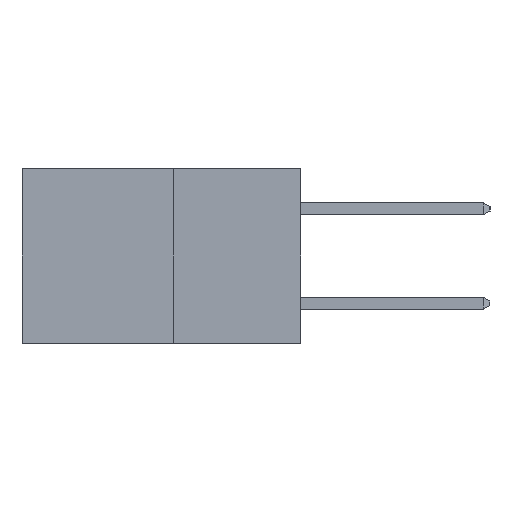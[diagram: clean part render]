
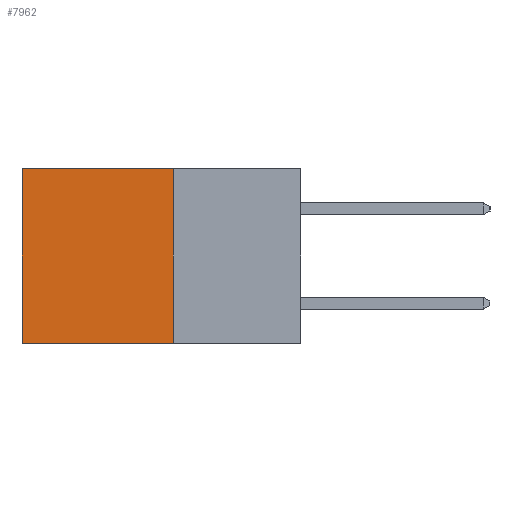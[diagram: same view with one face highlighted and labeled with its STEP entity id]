
A CAD part, left-side view. The second image highlights one B-rep face of the part: STEP entity #7962.
In plain terms, the highlighted planar face has unit normal (-1, 0, 0).
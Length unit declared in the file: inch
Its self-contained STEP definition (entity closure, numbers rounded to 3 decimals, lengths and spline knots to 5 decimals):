
#38 = VERTEX_POINT ( 'NONE', #3453 ) ;
#79 = DIRECTION ( 'NONE',  ( 0., 0., -1. ) ) ;
#374 = FACE_OUTER_BOUND ( 'NONE', #5023, .T. ) ;
#491 = VERTEX_POINT ( 'NONE', #4147 ) ;
#562 = DIRECTION ( 'NONE',  ( 1., 0., 0. ) ) ;
#1275 = VERTEX_POINT ( 'NONE', #5590 ) ;
#1349 = VECTOR ( 'NONE', #2227, 39.37008 ) ;
#1377 = DIRECTION ( 'NONE',  ( 0., 1., 0. ) ) ;
#1500 = CARTESIAN_POINT ( 'NONE',  ( 0.277, 0.27, -0.37 ) ) ;
#1899 = LINE ( 'NONE', #4761, #6907 ) ;
#2227 = DIRECTION ( 'NONE',  ( 0., 0., -1. ) ) ;
#2741 = VECTOR ( 'NONE', #5243, 39.37008 ) ;
#3453 = CARTESIAN_POINT ( 'NONE',  ( 0.277, 0.59, -0.37 ) ) ;
#3715 = EDGE_CURVE ( 'NONE', #1275, #38, #5634, .T. ) ;
#4147 = CARTESIAN_POINT ( 'NONE',  ( 0.277, 0.27, 0. ) ) ;
#4284 = VERTEX_POINT ( 'NONE', #6967 ) ;
#4662 = LINE ( 'NONE', #8142, #2741 ) ;
#4761 = CARTESIAN_POINT ( 'NONE',  ( 0.277, 0.27, 0. ) ) ;
#5023 = EDGE_LOOP ( 'NONE', ( #6057, #6078, #6053, #8007 ) ) ;
#5243 = DIRECTION ( 'NONE',  ( 0., 1., 0. ) ) ;
#5273 = DIRECTION ( 'NONE',  ( 0., 0., -1. ) ) ;
#5459 = AXIS2_PLACEMENT_3D ( 'NONE', #8164, #562, #5273 ) ;
#5590 = CARTESIAN_POINT ( 'NONE',  ( 0.277, 0.59, 0. ) ) ;
#5634 = LINE ( 'NONE', #7241, #7002 ) ;
#6053 = ORIENTED_EDGE ( 'NONE', *, *, #6471, .F. ) ;
#6057 = ORIENTED_EDGE ( 'NONE', *, *, #3715, .T. ) ;
#6078 = ORIENTED_EDGE ( 'NONE', *, *, #6213, .F. ) ;
#6213 = EDGE_CURVE ( 'NONE', #4284, #38, #4662, .T. ) ;
#6471 = EDGE_CURVE ( 'NONE', #491, #4284, #6479, .T. ) ;
#6479 = LINE ( 'NONE', #1500, #1349 ) ;
#6907 = VECTOR ( 'NONE', #1377, 39.37008 ) ;
#6967 = CARTESIAN_POINT ( 'NONE',  ( 0.277, 0.27, -0.37 ) ) ;
#7002 = VECTOR ( 'NONE', #79, 39.37008 ) ;
#7017 = PLANE ( 'NONE',  #5459 ) ;
#7241 = CARTESIAN_POINT ( 'NONE',  ( 0.277, 0.59, -0.37 ) ) ;
#7962 = ADVANCED_FACE ( 'NONE', ( #374 ), #7017, .F. ) ;
#8007 = ORIENTED_EDGE ( 'NONE', *, *, #8046, .T. ) ;
#8046 = EDGE_CURVE ( 'NONE', #491, #1275, #1899, .T. ) ;
#8142 = CARTESIAN_POINT ( 'NONE',  ( 0.277, 0.27, -0.37 ) ) ;
#8164 = CARTESIAN_POINT ( 'NONE',  ( 0.277, 0.27, -0.37 ) ) ;
